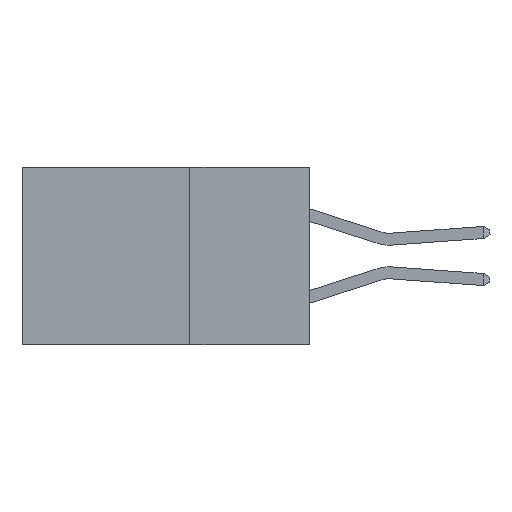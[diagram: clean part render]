
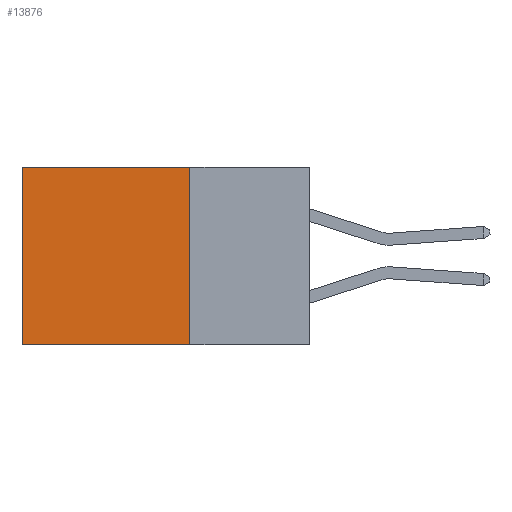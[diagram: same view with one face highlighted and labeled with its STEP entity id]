
A CAD part, left-side view. The second image highlights one B-rep face of the part: STEP entity #13876.
In plain terms, the highlighted planar face has unit normal (-1, 0, 0).
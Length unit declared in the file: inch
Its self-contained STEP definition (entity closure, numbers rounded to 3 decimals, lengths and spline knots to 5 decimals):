
#1067 = DIRECTION ( 'NONE',  ( 0., 1., 0. ) ) ;
#1298 = LINE ( 'NONE', #9743, #10421 ) ;
#2196 = LINE ( 'NONE', #9416, #14403 ) ;
#2879 = EDGE_LOOP ( 'NONE', ( #12986, #10894, #4557, #5335 ) ) ;
#2904 = CARTESIAN_POINT ( 'NONE',  ( 0.298, 0.25, -0.37 ) ) ;
#3049 = DIRECTION ( 'NONE',  ( 0., 0., -1. ) ) ;
#3519 = EDGE_CURVE ( 'NONE', #14805, #7717, #2196, .T. ) ;
#3820 = EDGE_CURVE ( 'NONE', #6487, #14805, #1298, .T. ) ;
#3878 = CARTESIAN_POINT ( 'NONE',  ( 0.298, 0.25, 0. ) ) ;
#4557 = ORIENTED_EDGE ( 'NONE', *, *, #14203, .F. ) ;
#5078 = DIRECTION ( 'NONE',  ( 1., 0., 0. ) ) ;
#5335 = ORIENTED_EDGE ( 'NONE', *, *, #3820, .T. ) ;
#5656 = CARTESIAN_POINT ( 'NONE',  ( 0.298, 0.6, 0. ) ) ;
#5782 = VERTEX_POINT ( 'NONE', #2904 ) ;
#5935 = LINE ( 'NONE', #6868, #11963 ) ;
#6487 = VERTEX_POINT ( 'NONE', #15050 ) ;
#6868 = CARTESIAN_POINT ( 'NONE',  ( 0.298, 0.25, 0. ) ) ;
#7600 = DIRECTION ( 'NONE',  ( 0., 1., 0. ) ) ;
#7717 = VERTEX_POINT ( 'NONE', #11197 ) ;
#8050 = AXIS2_PLACEMENT_3D ( 'NONE', #3878, #5078, #13384 ) ;
#8183 = CARTESIAN_POINT ( 'NONE',  ( 0.298, 0.25, -0.37 ) ) ;
#8503 = FACE_OUTER_BOUND ( 'NONE', #2879, .T. ) ;
#8709 = VECTOR ( 'NONE', #1067, 39.37008 ) ;
#9416 = CARTESIAN_POINT ( 'NONE',  ( 0.298, 0.6, 0. ) ) ;
#9743 = CARTESIAN_POINT ( 'NONE',  ( 0.298, 0.25, 0. ) ) ;
#10421 = VECTOR ( 'NONE', #7600, 39.37008 ) ;
#10894 = ORIENTED_EDGE ( 'NONE', *, *, #13626, .F. ) ;
#11035 = PLANE ( 'NONE',  #8050 ) ;
#11197 = CARTESIAN_POINT ( 'NONE',  ( 0.298, 0.6, -0.37 ) ) ;
#11963 = VECTOR ( 'NONE', #13967, 39.37008 ) ;
#12986 = ORIENTED_EDGE ( 'NONE', *, *, #3519, .T. ) ;
#13384 = DIRECTION ( 'NONE',  ( 0., 0., -1. ) ) ;
#13626 = EDGE_CURVE ( 'NONE', #5782, #7717, #14858, .T. ) ;
#13876 = ADVANCED_FACE ( 'NONE', ( #8503 ), #11035, .F. ) ;
#13967 = DIRECTION ( 'NONE',  ( 0., 0., -1. ) ) ;
#14203 = EDGE_CURVE ( 'NONE', #6487, #5782, #5935, .T. ) ;
#14403 = VECTOR ( 'NONE', #3049, 39.37008 ) ;
#14805 = VERTEX_POINT ( 'NONE', #5656 ) ;
#14858 = LINE ( 'NONE', #8183, #8709 ) ;
#15050 = CARTESIAN_POINT ( 'NONE',  ( 0.298, 0.25, 0. ) ) ;
